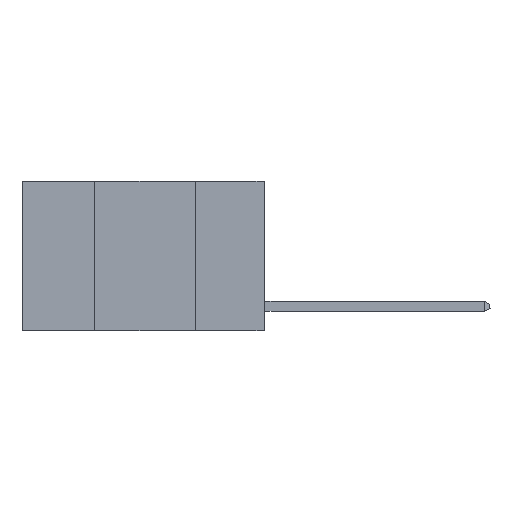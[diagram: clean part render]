
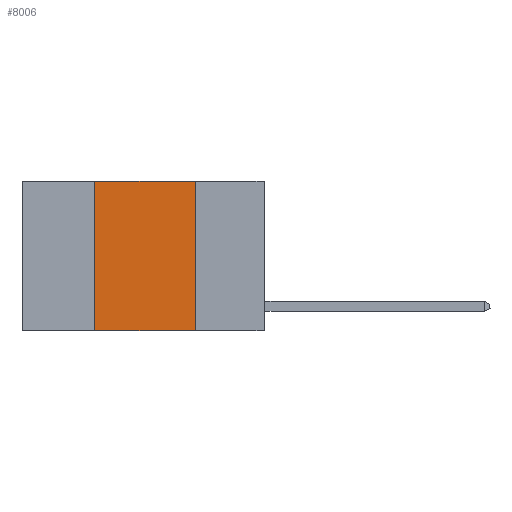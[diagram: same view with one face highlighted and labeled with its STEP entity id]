
A CAD part, left-side view. The second image highlights one B-rep face of the part: STEP entity #8006.
In plain terms, the highlighted planar face has unit normal (-1, 0, 0).
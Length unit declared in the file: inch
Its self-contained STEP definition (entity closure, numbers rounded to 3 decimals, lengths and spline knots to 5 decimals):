
#182 = EDGE_CURVE ( 'NONE', #7358, #9701, #13781, .T. ) ;
#289 = DIRECTION ( 'NONE',  ( 0., -1., 0. ) ) ;
#426 = EDGE_CURVE ( 'NONE', #4791, #9701, #9227, .T. ) ;
#1313 = VERTEX_POINT ( 'NONE', #11708 ) ;
#3046 = EDGE_LOOP ( 'NONE', ( #10837, #14341, #7858, #4661 ) ) ;
#3261 = CARTESIAN_POINT ( 'NONE',  ( 0., 0.17, -0.37 ) ) ;
#3686 = DIRECTION ( 'NONE',  ( 1., 0., 0. ) ) ;
#4371 = CARTESIAN_POINT ( 'NONE',  ( 0., 0.6, 0. ) ) ;
#4540 = CARTESIAN_POINT ( 'NONE',  ( 0., 0.42, -0.37 ) ) ;
#4577 = VECTOR ( 'NONE', #16016, 39.37008 ) ;
#4661 = ORIENTED_EDGE ( 'NONE', *, *, #426, .T. ) ;
#4791 = VERTEX_POINT ( 'NONE', #4540 ) ;
#5576 = VECTOR ( 'NONE', #8021, 39.37008 ) ;
#5599 = LINE ( 'NONE', #4371, #15888 ) ;
#6303 = CARTESIAN_POINT ( 'NONE',  ( 0., 0.17, 0. ) ) ;
#7358 = VERTEX_POINT ( 'NONE', #6303 ) ;
#7858 = ORIENTED_EDGE ( 'NONE', *, *, #17475, .F. ) ;
#7896 = CARTESIAN_POINT ( 'NONE',  ( 0., 0.6, -0.37 ) ) ;
#8006 = ADVANCED_FACE ( 'NONE', ( #13954 ), #11819, .F. ) ;
#8021 = DIRECTION ( 'NONE',  ( 0., -1., 0. ) ) ;
#8190 = LINE ( 'NONE', #15966, #4577 ) ;
#8421 = DIRECTION ( 'NONE',  ( 0., 0., -1. ) ) ;
#9227 = LINE ( 'NONE', #7896, #5576 ) ;
#9499 = AXIS2_PLACEMENT_3D ( 'NONE', #17055, #3686, #13138 ) ;
#9701 = VERTEX_POINT ( 'NONE', #3261 ) ;
#9869 = VECTOR ( 'NONE', #8421, 39.37008 ) ;
#10837 = ORIENTED_EDGE ( 'NONE', *, *, #182, .F. ) ;
#11708 = CARTESIAN_POINT ( 'NONE',  ( 0., 0.42, 0. ) ) ;
#11819 = PLANE ( 'NONE',  #9499 ) ;
#12879 = EDGE_CURVE ( 'NONE', #1313, #7358, #5599, .T. ) ;
#13138 = DIRECTION ( 'NONE',  ( 0., 0., -1. ) ) ;
#13781 = LINE ( 'NONE', #16055, #9869 ) ;
#13954 = FACE_OUTER_BOUND ( 'NONE', #3046, .T. ) ;
#14341 = ORIENTED_EDGE ( 'NONE', *, *, #12879, .F. ) ;
#15888 = VECTOR ( 'NONE', #289, 39.37008 ) ;
#15966 = CARTESIAN_POINT ( 'NONE',  ( 0., 0.42, 0. ) ) ;
#16016 = DIRECTION ( 'NONE',  ( 0., 0., 1. ) ) ;
#16055 = CARTESIAN_POINT ( 'NONE',  ( 0., 0.17, 0. ) ) ;
#17055 = CARTESIAN_POINT ( 'NONE',  ( 0., 0.6, 0. ) ) ;
#17475 = EDGE_CURVE ( 'NONE', #4791, #1313, #8190, .T. ) ;
